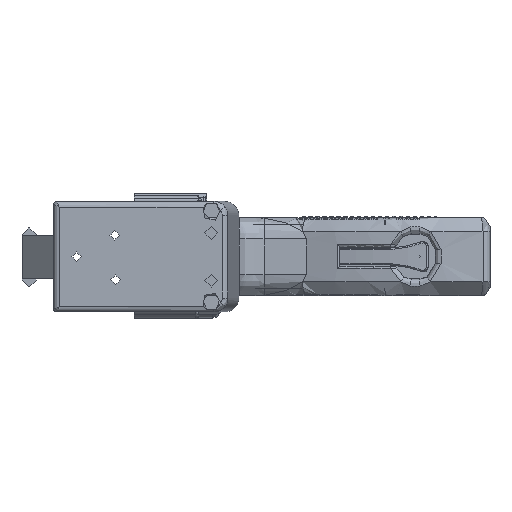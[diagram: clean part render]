
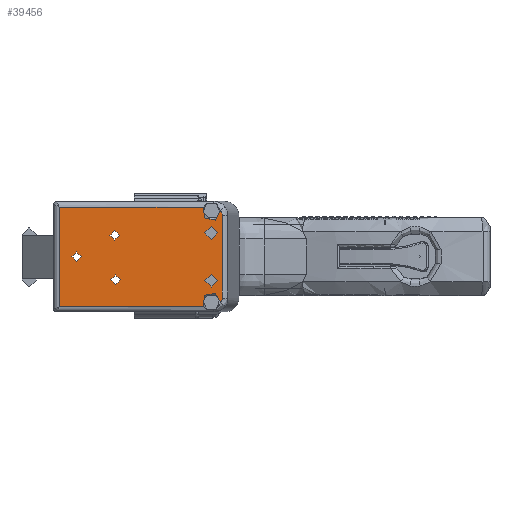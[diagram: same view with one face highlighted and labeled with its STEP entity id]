
A CAD part, left-side view. The second image highlights one B-rep face of the part: STEP entity #39456.
In plain terms, the highlighted planar face has unit normal (-1, 0, 0).
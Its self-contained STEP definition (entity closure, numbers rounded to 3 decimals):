
#550=FACE_BOUND('',#8182,.T.);
#551=FACE_BOUND('',#8183,.T.);
#552=FACE_BOUND('',#8184,.T.);
#553=FACE_BOUND('',#8185,.T.);
#554=FACE_BOUND('',#8186,.T.);
#729=ELLIPSE('',#43400,3.002,3.);
#731=ELLIPSE('',#43406,3.002,3.);
#3331=PLANE('',#43535);
#5648=FACE_OUTER_BOUND('',#8181,.T.);
#8181=EDGE_LOOP('',(#35792,#35793,#35794,#35795,#35796,#35797,#35798,#35799));
#8182=EDGE_LOOP('',(#35800));
#8183=EDGE_LOOP('',(#35801));
#8184=EDGE_LOOP('',(#35802));
#8185=EDGE_LOOP('',(#35803));
#8186=EDGE_LOOP('',(#35804));
#10488=LINE('',#215280,#12809);
#10489=LINE('',#215311,#12810);
#10547=LINE('',#216463,#12868);
#10561=LINE('',#216829,#12882);
#12809=VECTOR('',#53495,10.);
#12810=VECTOR('',#53506,10.);
#12868=VECTOR('',#53756,10.);
#12882=VECTOR('',#53846,10.);
#14937=CIRCLE('',#43388,1.75);
#14938=CIRCLE('',#43390,1.75);
#14939=CIRCLE('',#43392,1.7);
#14940=CIRCLE('',#43394,2.35);
#14941=CIRCLE('',#43396,2.35);
#14982=CIRCLE('',#43536,3.366);
#14983=CIRCLE('',#43537,3.366);
#18414=VERTEX_POINT('',#214986);
#18440=VERTEX_POINT('',#215258);
#18441=VERTEX_POINT('',#215262);
#18442=VERTEX_POINT('',#215266);
#18443=VERTEX_POINT('',#215270);
#18444=VERTEX_POINT('',#215274);
#18445=VERTEX_POINT('',#215278);
#18447=VERTEX_POINT('',#215302);
#18448=VERTEX_POINT('',#215304);
#18450=VERTEX_POINT('',#215310);
#18451=VERTEX_POINT('',#215334);
#18528=VERTEX_POINT('',#216454);
#18549=VERTEX_POINT('',#216827);
#24178=EDGE_CURVE('',#18440,#18440,#14937,.T.);
#24180=EDGE_CURVE('',#18441,#18441,#14938,.T.);
#24181=EDGE_CURVE('',#18442,#18442,#14939,.T.);
#24183=EDGE_CURVE('',#18443,#18443,#14940,.T.);
#24185=EDGE_CURVE('',#18444,#18444,#14941,.T.);
#24188=EDGE_CURVE('',#18414,#18445,#10488,.T.);
#24190=EDGE_CURVE('',#18447,#18448,#729,.T.);
#24193=EDGE_CURVE('',#18448,#18450,#10489,.T.);
#24197=EDGE_CURVE('',#18450,#18451,#731,.T.);
#24340=EDGE_CURVE('',#18528,#18414,#10547,.T.);
#24383=EDGE_CURVE('',#18528,#18451,#14982,.T.);
#24384=EDGE_CURVE('',#18447,#18549,#14983,.T.);
#24385=EDGE_CURVE('',#18445,#18549,#10561,.T.);
#35792=ORIENTED_EDGE('',*,*,#24340,.F.);
#35793=ORIENTED_EDGE('',*,*,#24383,.T.);
#35794=ORIENTED_EDGE('',*,*,#24197,.F.);
#35795=ORIENTED_EDGE('',*,*,#24193,.F.);
#35796=ORIENTED_EDGE('',*,*,#24190,.F.);
#35797=ORIENTED_EDGE('',*,*,#24384,.T.);
#35798=ORIENTED_EDGE('',*,*,#24385,.F.);
#35799=ORIENTED_EDGE('',*,*,#24188,.F.);
#35800=ORIENTED_EDGE('',*,*,#24185,.T.);
#35801=ORIENTED_EDGE('',*,*,#24183,.T.);
#35802=ORIENTED_EDGE('',*,*,#24181,.T.);
#35803=ORIENTED_EDGE('',*,*,#24180,.T.);
#35804=ORIENTED_EDGE('',*,*,#24178,.T.);
#39456=ADVANCED_FACE('',(#5648,#550,#551,#552,#553,#554),#3331,.T.);
#43388=AXIS2_PLACEMENT_3D('',#215260,#53469,#53470);
#43390=AXIS2_PLACEMENT_3D('',#215264,#53474,#53475);
#43392=AXIS2_PLACEMENT_3D('',#215267,#53478,#53479);
#43394=AXIS2_PLACEMENT_3D('',#215271,#53483,#53484);
#43396=AXIS2_PLACEMENT_3D('',#215275,#53488,#53489);
#43400=AXIS2_PLACEMENT_3D('',#215305,#53498,#53499);
#43406=AXIS2_PLACEMENT_3D('',#215336,#53512,#53513);
#43535=AXIS2_PLACEMENT_3D('',#216825,#53840,#53841);
#43536=AXIS2_PLACEMENT_3D('',#216826,#53842,#53843);
#43537=AXIS2_PLACEMENT_3D('',#216828,#53844,#53845);
#53469=DIRECTION('center_axis',(1.,0.,0.));
#53470=DIRECTION('ref_axis',(0.,1.,0.));
#53474=DIRECTION('center_axis',(1.,0.,0.));
#53475=DIRECTION('ref_axis',(0.,1.,0.));
#53478=DIRECTION('center_axis',(1.,0.,0.));
#53479=DIRECTION('ref_axis',(0.,0.,1.));
#53483=DIRECTION('center_axis',(1.,0.,0.));
#53484=DIRECTION('ref_axis',(0.,1.,0.));
#53488=DIRECTION('center_axis',(1.,0.,0.));
#53489=DIRECTION('ref_axis',(0.,1.,0.));
#53495=DIRECTION('',(0.,0.,1.));
#53498=DIRECTION('center_axis',(1.,0.,0.));
#53499=DIRECTION('ref_axis',(0.,-1.,0.));
#53506=DIRECTION('',(0.,0.,-1.));
#53512=DIRECTION('center_axis',(1.,0.,0.));
#53513=DIRECTION('ref_axis',(0.,-1.,0.));
#53756=DIRECTION('',(0.,1.,0.));
#53840=DIRECTION('center_axis',(-1.,0.,0.));
#53841=DIRECTION('ref_axis',(0.,0.,1.));
#53842=DIRECTION('center_axis',(1.,0.,0.));
#53843=DIRECTION('ref_axis',(0.,-1.,0.));
#53844=DIRECTION('center_axis',(1.,0.,0.));
#53845=DIRECTION('ref_axis',(0.,-1.,0.));
#53846=DIRECTION('',(0.,-1.,0.));
#214986=CARTESIAN_POINT('',(-241.376,39.25,-3.08));
#215258=CARTESIAN_POINT('',(-241.376,17.264,6.52));
#215260=CARTESIAN_POINT('Origin',(-241.376,19.014,6.52));
#215262=CARTESIAN_POINT('',(-241.376,17.554,22.493));
#215264=CARTESIAN_POINT('Origin',(-241.376,19.304,22.493));
#215266=CARTESIAN_POINT('',(-241.376,33.049,13.096));
#215267=CARTESIAN_POINT('Origin',(-241.376,33.049,14.796));
#215270=CARTESIAN_POINT('',(-241.376,-17.785,6.222));
#215271=CARTESIAN_POINT('Origin',(-241.376,-15.435,6.222));
#215274=CARTESIAN_POINT('',(-241.376,-17.785,23.367));
#215275=CARTESIAN_POINT('Origin',(-241.376,-15.435,23.367));
#215278=CARTESIAN_POINT('',(-241.376,39.25,32.671));
#215280=CARTESIAN_POINT('',(-241.376,39.25,24.733));
#215302=CARTESIAN_POINT('',(-241.376,-18.813,31.415));
#215304=CARTESIAN_POINT('',(-241.376,-19.372,29.671));
#215305=CARTESIAN_POINT('Origin',(-241.376,-16.37,29.671));
#215310=CARTESIAN_POINT('',(-241.376,-19.372,-0.08));
#215311=CARTESIAN_POINT('',(-241.376,-19.372,24.733));
#215334=CARTESIAN_POINT('',(-241.376,-18.809,-1.829));
#215336=CARTESIAN_POINT('Origin',(-241.376,-16.37,-0.08));
#216454=CARTESIAN_POINT('',(-241.376,-12.565,-3.08));
#216463=CARTESIAN_POINT('',(-241.376,6.156,-3.08));
#216825=CARTESIAN_POINT('Origin',(-241.376,7.049,14.796));
#216826=CARTESIAN_POINT('Origin',(-241.376,-15.473,-1.385));
#216827=CARTESIAN_POINT('',(-241.376,-12.552,32.671));
#216828=CARTESIAN_POINT('Origin',(-241.376,-15.473,31.));
#216829=CARTESIAN_POINT('',(-241.376,-1.289,32.671));
